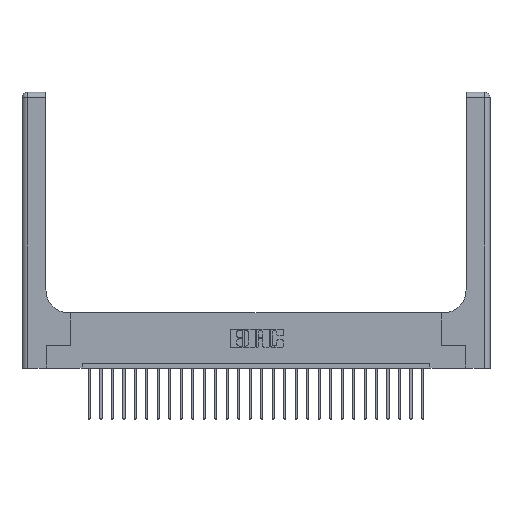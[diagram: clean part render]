
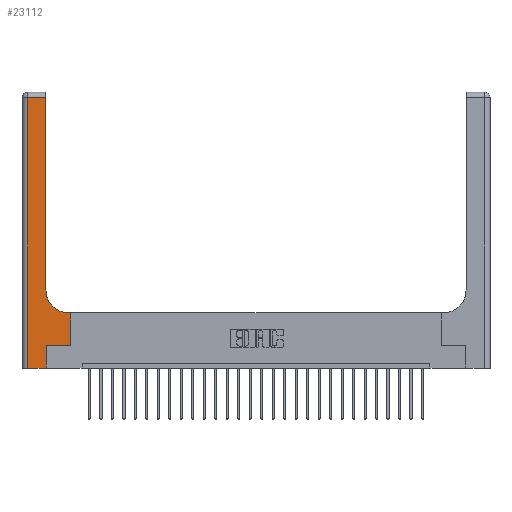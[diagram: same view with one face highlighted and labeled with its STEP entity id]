
A CAD part, top view. The second image highlights one B-rep face of the part: STEP entity #23112.
In plain terms, the highlighted planar face has unit normal (0, 0, 1).
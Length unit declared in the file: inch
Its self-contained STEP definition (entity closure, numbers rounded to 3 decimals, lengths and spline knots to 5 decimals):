
#217 = ORIENTED_EDGE ( 'NONE', *, *, #19806, .T. ) ;
#242 = VERTEX_POINT ( 'NONE', #17006 ) ;
#1061 = DIRECTION ( 'NONE',  ( 1., 0., 0. ) ) ;
#1292 = EDGE_CURVE ( 'NONE', #12008, #17517, #10362, .T. ) ;
#1401 = CARTESIAN_POINT ( 'NONE',  ( 0.265, 0.25, 0.37 ) ) ;
#1698 = DIRECTION ( 'NONE',  ( 0., 0., -1. ) ) ;
#1877 = VECTOR ( 'NONE', #13827, 39.37008 ) ;
#3087 = VERTEX_POINT ( 'NONE', #15508 ) ;
#3795 = CARTESIAN_POINT ( 'NONE',  ( 0.51, 0.6, 0.37 ) ) ;
#4056 = LINE ( 'NONE', #18038, #10726 ) ;
#4206 = AXIS2_PLACEMENT_3D ( 'NONE', #25498, #1698, #23535 ) ;
#4212 = CARTESIAN_POINT ( 'NONE',  ( 0.265, 0., 0.37 ) ) ;
#4223 = ORIENTED_EDGE ( 'NONE', *, *, #1292, .T. ) ;
#4305 = CARTESIAN_POINT ( 'NONE',  ( 0.26, 2.94, 0.37 ) ) ;
#4428 = CARTESIAN_POINT ( 'NONE',  ( 0.26, 0.6, 0.37 ) ) ;
#4534 = VERTEX_POINT ( 'NONE', #14889 ) ;
#4766 = LINE ( 'NONE', #24622, #10494 ) ;
#4883 = EDGE_CURVE ( 'NONE', #242, #12008, #10898, .T. ) ;
#5055 = CIRCLE ( 'NONE', #4206, 0.25 ) ;
#5133 = LINE ( 'NONE', #12986, #16189 ) ;
#5339 = ORIENTED_EDGE ( 'NONE', *, *, #24566, .T. ) ;
#5444 = VECTOR ( 'NONE', #22642, 39.37008 ) ;
#7094 = CARTESIAN_POINT ( 'NONE',  ( 0., 0., 0.37 ) ) ;
#7267 = FACE_OUTER_BOUND ( 'NONE', #19905, .T. ) ;
#7887 = EDGE_CURVE ( 'NONE', #21428, #12850, #13858, .T. ) ;
#7917 = DIRECTION ( 'NONE',  ( -1., 0., 0. ) ) ;
#7970 = CARTESIAN_POINT ( 'NONE',  ( 0.26, 3., 0.37 ) ) ;
#8046 = EDGE_CURVE ( 'NONE', #3087, #9744, #16332, .T. ) ;
#8456 = VECTOR ( 'NONE', #21838, 39.37008 ) ;
#9366 = PLANE ( 'NONE',  #22130 ) ;
#9744 = VERTEX_POINT ( 'NONE', #3795 ) ;
#10362 = LINE ( 'NONE', #4212, #5444 ) ;
#10494 = VECTOR ( 'NONE', #16053, 39.37008 ) ;
#10726 = VECTOR ( 'NONE', #16091, 39.37008 ) ;
#10831 = ORIENTED_EDGE ( 'NONE', *, *, #8046, .T. ) ;
#10898 = LINE ( 'NONE', #7094, #24365 ) ;
#10933 = EDGE_CURVE ( 'NONE', #12850, #4534, #4056, .T. ) ;
#11484 = CARTESIAN_POINT ( 'NONE',  ( 0.265, 0.25, 0.37 ) ) ;
#12008 = VERTEX_POINT ( 'NONE', #20072 ) ;
#12850 = VERTEX_POINT ( 'NONE', #4305 ) ;
#12853 = DIRECTION ( 'NONE',  ( 0., 1., 0. ) ) ;
#12986 = CARTESIAN_POINT ( 'NONE',  ( 0.528, 0.25, 0.37 ) ) ;
#13116 = ORIENTED_EDGE ( 'NONE', *, *, #10933, .T. ) ;
#13602 = CARTESIAN_POINT ( 'NONE',  ( 0.528, 0.25, 0.37 ) ) ;
#13827 = DIRECTION ( 'NONE',  ( 1., 0., 0. ) ) ;
#13858 = LINE ( 'NONE', #7970, #8456 ) ;
#14629 = CARTESIAN_POINT ( 'NONE',  ( 0.26, 0.85, 0.37 ) ) ;
#14889 = CARTESIAN_POINT ( 'NONE',  ( 0.06, 2.94, 0.37 ) ) ;
#15508 = CARTESIAN_POINT ( 'NONE',  ( 0.528, 0.6, 0.37 ) ) ;
#16053 = DIRECTION ( 'NONE',  ( 0., -1., 0. ) ) ;
#16091 = DIRECTION ( 'NONE',  ( -1., 0., 0. ) ) ;
#16189 = VECTOR ( 'NONE', #12853, 39.37008 ) ;
#16332 = LINE ( 'NONE', #4428, #22645 ) ;
#16379 = ORIENTED_EDGE ( 'NONE', *, *, #24067, .T. ) ;
#16446 = ORIENTED_EDGE ( 'NONE', *, *, #7887, .T. ) ;
#17006 = CARTESIAN_POINT ( 'NONE',  ( 0.06, 0., 0.37 ) ) ;
#17234 = LINE ( 'NONE', #1401, #1877 ) ;
#17424 = EDGE_CURVE ( 'NONE', #17517, #20445, #17234, .T. ) ;
#17517 = VERTEX_POINT ( 'NONE', #11484 ) ;
#18038 = CARTESIAN_POINT ( 'NONE',  ( 0., 2.94, 0.37 ) ) ;
#19806 = EDGE_CURVE ( 'NONE', #20445, #3087, #5133, .T. ) ;
#19905 = EDGE_LOOP ( 'NONE', ( #16446, #13116, #5339, #23082, #4223, #22243, #217, #10831, #16379 ) ) ;
#20072 = CARTESIAN_POINT ( 'NONE',  ( 0.265, 0., 0.37 ) ) ;
#20190 = DIRECTION ( 'NONE',  ( 0., 0., -1. ) ) ;
#20445 = VERTEX_POINT ( 'NONE', #13602 ) ;
#21428 = VERTEX_POINT ( 'NONE', #14629 ) ;
#21838 = DIRECTION ( 'NONE',  ( 0., 1., 0. ) ) ;
#22130 = AXIS2_PLACEMENT_3D ( 'NONE', #23599, #20190, #7917 ) ;
#22243 = ORIENTED_EDGE ( 'NONE', *, *, #17424, .T. ) ;
#22642 = DIRECTION ( 'NONE',  ( 0., 1., 0. ) ) ;
#22645 = VECTOR ( 'NONE', #24541, 39.37008 ) ;
#23082 = ORIENTED_EDGE ( 'NONE', *, *, #4883, .T. ) ;
#23112 = ADVANCED_FACE ( 'NONE', ( #7267 ), #9366, .F. ) ;
#23535 = DIRECTION ( 'NONE',  ( 1., 0., 0. ) ) ;
#23599 = CARTESIAN_POINT ( 'NONE',  ( 0., 3., 0.37 ) ) ;
#24067 = EDGE_CURVE ( 'NONE', #9744, #21428, #5055, .T. ) ;
#24365 = VECTOR ( 'NONE', #1061, 39.37008 ) ;
#24541 = DIRECTION ( 'NONE',  ( -1., 0., 0. ) ) ;
#24566 = EDGE_CURVE ( 'NONE', #4534, #242, #4766, .T. ) ;
#24622 = CARTESIAN_POINT ( 'NONE',  ( 0.06, 3., 0.37 ) ) ;
#25498 = CARTESIAN_POINT ( 'NONE',  ( 0.51, 0.85, 0.37 ) ) ;
